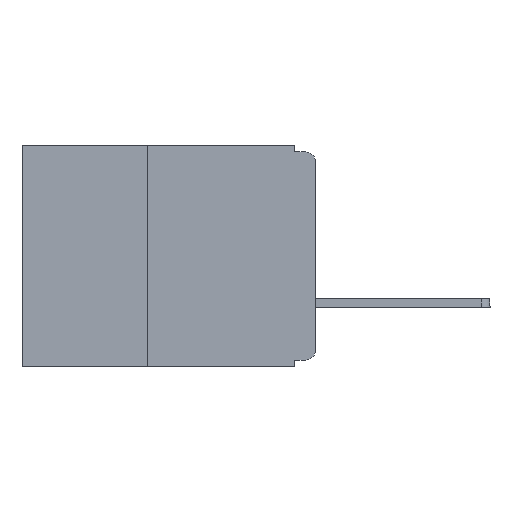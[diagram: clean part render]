
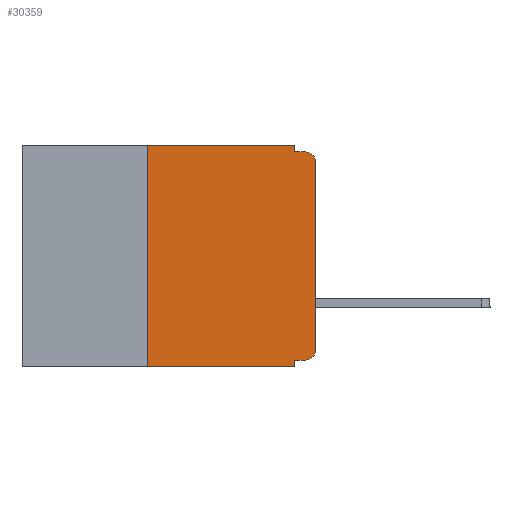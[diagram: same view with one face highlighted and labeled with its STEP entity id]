
A CAD part, left-side view. The second image highlights one B-rep face of the part: STEP entity #30359.
In plain terms, the highlighted planar face has unit normal (-1, 0, 0).
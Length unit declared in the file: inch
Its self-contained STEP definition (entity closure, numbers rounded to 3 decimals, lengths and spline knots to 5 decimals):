
#1133 = ORIENTED_EDGE ( 'NONE', *, *, #14275, .T. ) ;
#1241 = DIRECTION ( 'NONE',  ( 0., 0., -1. ) ) ;
#2456 = LINE ( 'NONE', #6250, #23742 ) ;
#3431 = EDGE_CURVE ( 'NONE', #23555, #16292, #20253, .T. ) ;
#3887 = ORIENTED_EDGE ( 'NONE', *, *, #20863, .F. ) ;
#4394 = VERTEX_POINT ( 'NONE', #6708 ) ;
#4626 = LINE ( 'NONE', #15685, #29968 ) ;
#4706 = VERTEX_POINT ( 'NONE', #29528 ) ;
#4872 = CARTESIAN_POINT ( 'NONE',  ( 0., 0.25, -0.33 ) ) ;
#5239 = DIRECTION ( 'NONE',  ( 0., 1., 0. ) ) ;
#5423 = CARTESIAN_POINT ( 'NONE',  ( 0., 0., -0.32 ) ) ;
#5832 = DIRECTION ( 'NONE',  ( 0., 0., -1. ) ) ;
#5850 = CARTESIAN_POINT ( 'NONE',  ( 0., 0.25, 0. ) ) ;
#6250 = CARTESIAN_POINT ( 'NONE',  ( 0., 0.031, 0. ) ) ;
#6269 = EDGE_CURVE ( 'NONE', #4394, #4706, #11986, .T. ) ;
#6273 = AXIS2_PLACEMENT_3D ( 'NONE', #8719, #16168, #1241 ) ;
#6316 = VERTEX_POINT ( 'NONE', #4872 ) ;
#6708 = CARTESIAN_POINT ( 'NONE',  ( 0., 0.015, -0.32 ) ) ;
#8172 = DIRECTION ( 'NONE',  ( 0., 0., -1. ) ) ;
#8201 = CARTESIAN_POINT ( 'NONE',  ( 0., 0.031, -0.01 ) ) ;
#8305 = VERTEX_POINT ( 'NONE', #23378 ) ;
#8307 = DIRECTION ( 'NONE',  ( -1., 0., 0. ) ) ;
#8347 = CARTESIAN_POINT ( 'NONE',  ( 0., 0.015, -0.025 ) ) ;
#8455 = LINE ( 'NONE', #22267, #14272 ) ;
#8690 = CARTESIAN_POINT ( 'NONE',  ( 0., 0., -0.01 ) ) ;
#8719 = CARTESIAN_POINT ( 'NONE',  ( 0., 0.437, 0. ) ) ;
#9993 = DIRECTION ( 'NONE',  ( 0., -1., 0. ) ) ;
#10552 = EDGE_CURVE ( 'NONE', #22928, #23555, #19217, .T. ) ;
#10880 = VECTOR ( 'NONE', #11167, 39.37008 ) ;
#11167 = DIRECTION ( 'NONE',  ( 0., -1., 0. ) ) ;
#11280 = EDGE_CURVE ( 'NONE', #24940, #23510, #2456, .T. ) ;
#11632 = CARTESIAN_POINT ( 'NONE',  ( 0., 0.031, 0. ) ) ;
#11986 = LINE ( 'NONE', #5423, #16232 ) ;
#12214 = ORIENTED_EDGE ( 'NONE', *, *, #27138, .F. ) ;
#12661 = CARTESIAN_POINT ( 'NONE',  ( 0., 0.015, -0.305 ) ) ;
#12783 = FACE_OUTER_BOUND ( 'NONE', #24568, .T. ) ;
#13611 = EDGE_CURVE ( 'NONE', #6316, #30841, #30804, .T. ) ;
#13719 = CARTESIAN_POINT ( 'NONE',  ( 0., 0.015, -0.01 ) ) ;
#14272 = VECTOR ( 'NONE', #9993, 39.37008 ) ;
#14275 = EDGE_CURVE ( 'NONE', #6316, #8305, #18234, .T. ) ;
#14934 = EDGE_CURVE ( 'NONE', #4706, #8305, #4626, .T. ) ;
#15070 = CARTESIAN_POINT ( 'NONE',  ( 0., 0., 0. ) ) ;
#15140 = DIRECTION ( 'NONE',  ( 0., 0., -1. ) ) ;
#15289 = AXIS2_PLACEMENT_3D ( 'NONE', #8347, #8307, #8172 ) ;
#15441 = ORIENTED_EDGE ( 'NONE', *, *, #26277, .T. ) ;
#15517 = CARTESIAN_POINT ( 'NONE',  ( 0., 0.437, -0.33 ) ) ;
#15685 = CARTESIAN_POINT ( 'NONE',  ( 0., 0.031, -0.33 ) ) ;
#16168 = DIRECTION ( 'NONE',  ( 1., 0., 0. ) ) ;
#16232 = VECTOR ( 'NONE', #5239, 39.37008 ) ;
#16292 = VERTEX_POINT ( 'NONE', #13719 ) ;
#16992 = AXIS2_PLACEMENT_3D ( 'NONE', #12661, #29733, #15140 ) ;
#17908 = CARTESIAN_POINT ( 'NONE',  ( 0., 0.25, -0.33 ) ) ;
#18066 = CARTESIAN_POINT ( 'NONE',  ( 0., 0., -0.305 ) ) ;
#18234 = LINE ( 'NONE', #15517, #23954 ) ;
#18682 = VECTOR ( 'NONE', #20395, 39.37008 ) ;
#19217 = LINE ( 'NONE', #15070, #31331 ) ;
#20253 = CIRCLE ( 'NONE', #15289, 0.015 ) ;
#20395 = DIRECTION ( 'NONE',  ( 0., 0., 1. ) ) ;
#20863 = EDGE_CURVE ( 'NONE', #23510, #16292, #23946, .T. ) ;
#21446 = ORIENTED_EDGE ( 'NONE', *, *, #6269, .F. ) ;
#21618 = CIRCLE ( 'NONE', #16992, 0.015 ) ;
#22267 = CARTESIAN_POINT ( 'NONE',  ( 0., 0.437, 0. ) ) ;
#22460 = ORIENTED_EDGE ( 'NONE', *, *, #14934, .F. ) ;
#22464 = DIRECTION ( 'NONE',  ( 0., 0., 1. ) ) ;
#22905 = DIRECTION ( 'NONE',  ( 0., -1., 0. ) ) ;
#22928 = VERTEX_POINT ( 'NONE', #18066 ) ;
#23378 = CARTESIAN_POINT ( 'NONE',  ( 0., 0.031, -0.33 ) ) ;
#23499 = DIRECTION ( 'NONE',  ( 0., 0., -1. ) ) ;
#23510 = VERTEX_POINT ( 'NONE', #8201 ) ;
#23555 = VERTEX_POINT ( 'NONE', #28582 ) ;
#23742 = VECTOR ( 'NONE', #23499, 39.37008 ) ;
#23946 = LINE ( 'NONE', #8690, #10880 ) ;
#23954 = VECTOR ( 'NONE', #22905, 39.37008 ) ;
#24014 = ORIENTED_EDGE ( 'NONE', *, *, #3431, .T. ) ;
#24520 = ORIENTED_EDGE ( 'NONE', *, *, #11280, .F. ) ;
#24568 = EDGE_LOOP ( 'NONE', ( #31808, #24014, #3887, #24520, #12214, #31824, #1133, #22460, #21446, #15441 ) ) ;
#24940 = VERTEX_POINT ( 'NONE', #11632 ) ;
#25852 = PLANE ( 'NONE',  #6273 ) ;
#26277 = EDGE_CURVE ( 'NONE', #4394, #22928, #21618, .T. ) ;
#27138 = EDGE_CURVE ( 'NONE', #30841, #24940, #8455, .T. ) ;
#28582 = CARTESIAN_POINT ( 'NONE',  ( 0., 0., -0.025 ) ) ;
#29528 = CARTESIAN_POINT ( 'NONE',  ( 0., 0.031, -0.32 ) ) ;
#29733 = DIRECTION ( 'NONE',  ( -1., 0., 0. ) ) ;
#29968 = VECTOR ( 'NONE', #5832, 39.37008 ) ;
#30359 = ADVANCED_FACE ( 'NONE', ( #12783 ), #25852, .F. ) ;
#30804 = LINE ( 'NONE', #17908, #18682 ) ;
#30841 = VERTEX_POINT ( 'NONE', #5850 ) ;
#31331 = VECTOR ( 'NONE', #22464, 39.37008 ) ;
#31808 = ORIENTED_EDGE ( 'NONE', *, *, #10552, .T. ) ;
#31824 = ORIENTED_EDGE ( 'NONE', *, *, #13611, .F. ) ;
